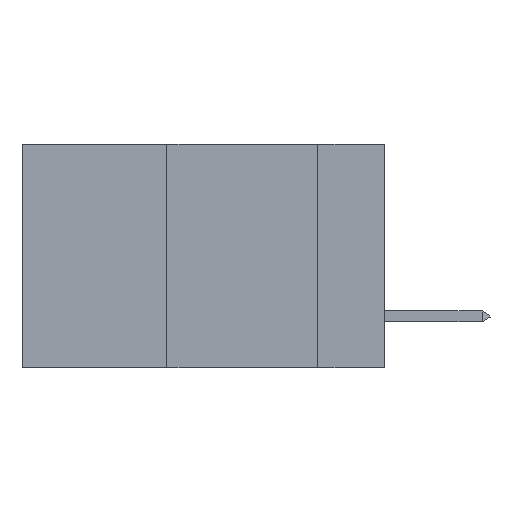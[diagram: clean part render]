
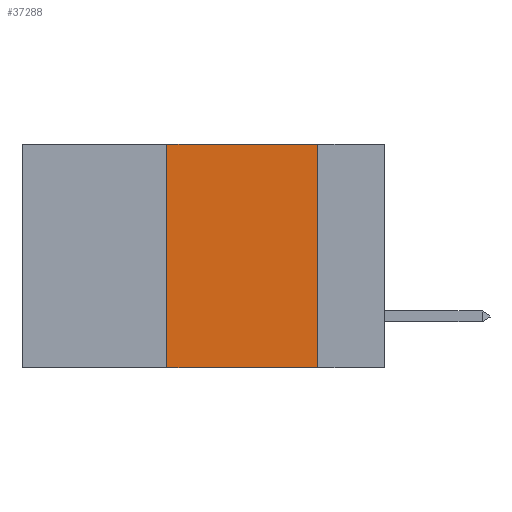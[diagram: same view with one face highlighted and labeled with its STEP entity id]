
A CAD part, left-side view. The second image highlights one B-rep face of the part: STEP entity #37288.
In plain terms, the highlighted planar face has unit normal (-1, 0, 0).
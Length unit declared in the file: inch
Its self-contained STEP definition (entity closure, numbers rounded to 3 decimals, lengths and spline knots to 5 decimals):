
#310 = VERTEX_POINT ( 'NONE', #8164 ) ;
#1425 = LINE ( 'NONE', #20198, #36038 ) ;
#2114 = VECTOR ( 'NONE', #31970, 39.37008 ) ;
#2701 = DIRECTION ( 'NONE',  ( 0., 0., -1. ) ) ;
#3154 = CARTESIAN_POINT ( 'NONE',  ( 0., 0.6, 0. ) ) ;
#3553 = VERTEX_POINT ( 'NONE', #8185 ) ;
#6994 = DIRECTION ( 'NONE',  ( 1., 0., 0. ) ) ;
#8164 = CARTESIAN_POINT ( 'NONE',  ( 0., 0.36, 0. ) ) ;
#8185 = CARTESIAN_POINT ( 'NONE',  ( 0., 0.11, -0.37 ) ) ;
#10134 = ORIENTED_EDGE ( 'NONE', *, *, #19147, .F. ) ;
#10278 = DIRECTION ( 'NONE',  ( 0., -1., 0. ) ) ;
#11131 = LINE ( 'NONE', #21201, #2114 ) ;
#11576 = CARTESIAN_POINT ( 'NONE',  ( 0., 0.36, -0.37 ) ) ;
#11888 = AXIS2_PLACEMENT_3D ( 'NONE', #3154, #6994, #33886 ) ;
#15287 = LINE ( 'NONE', #25696, #24776 ) ;
#15834 = EDGE_CURVE ( 'NONE', #44242, #3553, #15287, .T. ) ;
#16403 = EDGE_CURVE ( 'NONE', #310, #44242, #11131, .T. ) ;
#17301 = CARTESIAN_POINT ( 'NONE',  ( 0., 0.11, 0. ) ) ;
#19147 = EDGE_CURVE ( 'NONE', #47532, #310, #44601, .T. ) ;
#20088 = ORIENTED_EDGE ( 'NONE', *, *, #36521, .T. ) ;
#20198 = CARTESIAN_POINT ( 'NONE',  ( 0., 0.6, -0.37 ) ) ;
#21085 = DIRECTION ( 'NONE',  ( 0., 0., 1. ) ) ;
#21201 = CARTESIAN_POINT ( 'NONE',  ( 0., 0.6, 0. ) ) ;
#23442 = FACE_OUTER_BOUND ( 'NONE', #42316, .T. ) ;
#24776 = VECTOR ( 'NONE', #2701, 39.37008 ) ;
#25696 = CARTESIAN_POINT ( 'NONE',  ( 0., 0.11, 0. ) ) ;
#31970 = DIRECTION ( 'NONE',  ( 0., -1., 0. ) ) ;
#33886 = DIRECTION ( 'NONE',  ( 0., 0., -1. ) ) ;
#36038 = VECTOR ( 'NONE', #10278, 39.37008 ) ;
#36521 = EDGE_CURVE ( 'NONE', #47532, #3553, #1425, .T. ) ;
#37288 = ADVANCED_FACE ( 'NONE', ( #23442 ), #45495, .F. ) ;
#42316 = EDGE_LOOP ( 'NONE', ( #49061, #42917, #10134, #20088 ) ) ;
#42917 = ORIENTED_EDGE ( 'NONE', *, *, #16403, .F. ) ;
#44242 = VERTEX_POINT ( 'NONE', #17301 ) ;
#44601 = LINE ( 'NONE', #47261, #45679 ) ;
#45495 = PLANE ( 'NONE',  #11888 ) ;
#45679 = VECTOR ( 'NONE', #21085, 39.37008 ) ;
#47261 = CARTESIAN_POINT ( 'NONE',  ( 0., 0.36, 0. ) ) ;
#47532 = VERTEX_POINT ( 'NONE', #11576 ) ;
#49061 = ORIENTED_EDGE ( 'NONE', *, *, #15834, .F. ) ;
